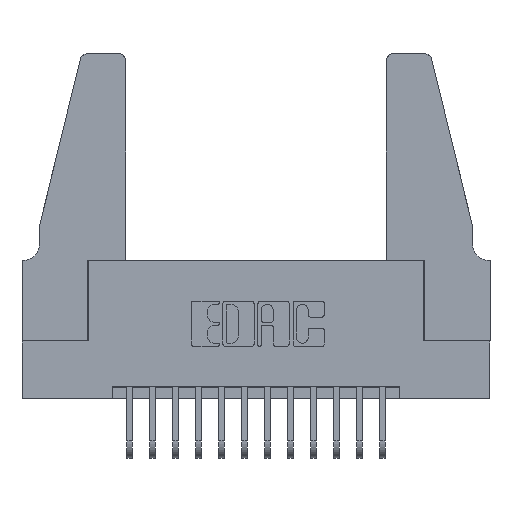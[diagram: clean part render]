
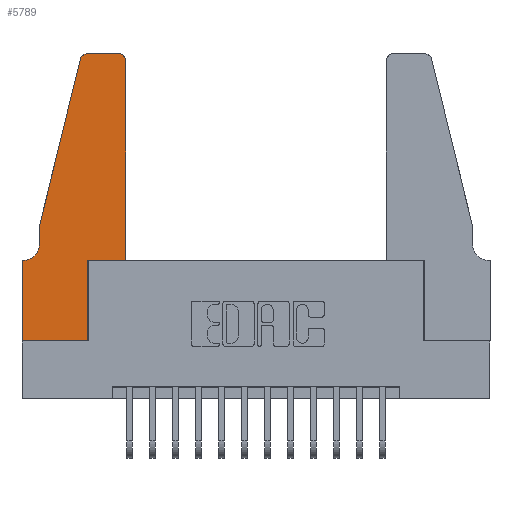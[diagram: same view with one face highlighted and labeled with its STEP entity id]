
A CAD part, top view. The second image highlights one B-rep face of the part: STEP entity #5789.
In plain terms, the highlighted planar face has unit normal (0, 0, 1).
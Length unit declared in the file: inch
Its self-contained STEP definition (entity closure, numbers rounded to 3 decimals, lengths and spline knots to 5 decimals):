
#34 = CARTESIAN_POINT ( 'NONE',  ( 0.4205, 1.22, 0.37 ) ) ;
#195 = EDGE_CURVE ( 'NONE', #236, #10536, #16336, .T. ) ;
#236 = VERTEX_POINT ( 'NONE', #4721 ) ;
#708 = ORIENTED_EDGE ( 'NONE', *, *, #14038, .T. ) ;
#716 = EDGE_CURVE ( 'NONE', #9279, #2787, #15521, .T. ) ;
#988 = EDGE_CURVE ( 'NONE', #12800, #6573, #12059, .T. ) ;
#1186 = DIRECTION ( 'NONE',  ( 0., 1., 0. ) ) ;
#1189 = CARTESIAN_POINT ( 'NONE',  ( 0.0755, 0.5, 0.37 ) ) ;
#1417 = DIRECTION ( 'NONE',  ( 1., 0., 0. ) ) ;
#1573 = CARTESIAN_POINT ( 'NONE',  ( 0., 0., 0.37 ) ) ;
#1578 = CARTESIAN_POINT ( 'NONE',  ( 0.284, 1.22, 0.37 ) ) ;
#1731 = LINE ( 'NONE', #1573, #8723 ) ;
#1789 = DIRECTION ( 'NONE',  ( 0., -1., 0. ) ) ;
#1883 = VECTOR ( 'NONE', #7935, 39.37008 ) ;
#2239 = ORIENTED_EDGE ( 'NONE', *, *, #7657, .T. ) ;
#2275 = EDGE_CURVE ( 'NONE', #6573, #14559, #14823, .T. ) ;
#2377 = FACE_OUTER_BOUND ( 'NONE', #6181, .T. ) ;
#2787 = VERTEX_POINT ( 'NONE', #11949 ) ;
#2985 = DIRECTION ( 'NONE',  ( 0., -1., 0. ) ) ;
#2988 = DIRECTION ( 'NONE',  ( 1., 0., 0. ) ) ;
#3435 = EDGE_CURVE ( 'NONE', #17210, #11579, #15969, .T. ) ;
#3526 = PLANE ( 'NONE',  #13169 ) ;
#3798 = DIRECTION ( 'NONE',  ( 1., 0., 0. ) ) ;
#4721 = CARTESIAN_POINT ( 'NONE',  ( 0.0755, 0.42, 0.37 ) ) ;
#4843 = DIRECTION ( 'NONE',  ( 0., 0., -1. ) ) ;
#4886 = CARTESIAN_POINT ( 'NONE',  ( 0.0055, 0.42, 0.37 ) ) ;
#4916 = VERTEX_POINT ( 'NONE', #16343 ) ;
#4931 = DIRECTION ( 'NONE',  ( 0., 0., 1. ) ) ;
#5191 = DIRECTION ( 'NONE',  ( -1., 0., 0. ) ) ;
#5255 = CARTESIAN_POINT ( 'NONE',  ( 0.4505, 1.22, 0.37 ) ) ;
#5608 = LINE ( 'NONE', #16929, #1883 ) ;
#5740 = CARTESIAN_POINT ( 'NONE',  ( 0.4205, 1.25, 0.37 ) ) ;
#5789 = ADVANCED_FACE ( 'NONE', ( #2377 ), #3526, .T. ) ;
#6181 = EDGE_LOOP ( 'NONE', ( #15195, #12189, #9197, #2239, #9609, #16388, #10016, #13382, #10435, #7247, #10819, #708 ) ) ;
#6261 = CARTESIAN_POINT ( 'NONE',  ( 0., 0.35, 0.37 ) ) ;
#6550 = CIRCLE ( 'NONE', #13140, 0.03 ) ;
#6573 = VERTEX_POINT ( 'NONE', #16811 ) ;
#6599 = CARTESIAN_POINT ( 'NONE',  ( 0., 0., 0.37 ) ) ;
#6627 = VECTOR ( 'NONE', #14822, 39.37008 ) ;
#6824 = DIRECTION ( 'NONE',  ( -0.239, -0.971, 0. ) ) ;
#6870 = CARTESIAN_POINT ( 'NONE',  ( 0., 0., 0.37 ) ) ;
#6939 = EDGE_CURVE ( 'NONE', #2787, #4916, #10712, .T. ) ;
#7191 = LINE ( 'NONE', #17166, #13725 ) ;
#7247 = ORIENTED_EDGE ( 'NONE', *, *, #988, .T. ) ;
#7657 = EDGE_CURVE ( 'NONE', #11044, #236, #10343, .T. ) ;
#7935 = DIRECTION ( 'NONE',  ( -1., 0., 0. ) ) ;
#8176 = VECTOR ( 'NONE', #11530, 39.37008 ) ;
#8723 = VECTOR ( 'NONE', #2985, 39.37008 ) ;
#9197 = ORIENTED_EDGE ( 'NONE', *, *, #9750, .T. ) ;
#9279 = VERTEX_POINT ( 'NONE', #5740 ) ;
#9481 = VERTEX_POINT ( 'NONE', #12821 ) ;
#9609 = ORIENTED_EDGE ( 'NONE', *, *, #195, .T. ) ;
#9732 = DIRECTION ( 'NONE',  ( 0., 0., 1. ) ) ;
#9750 = EDGE_CURVE ( 'NONE', #4916, #11044, #13837, .T. ) ;
#10016 = ORIENTED_EDGE ( 'NONE', *, *, #13219, .T. ) ;
#10085 = CARTESIAN_POINT ( 'NONE',  ( 0.0755, 0.5, 0.37 ) ) ;
#10343 = LINE ( 'NONE', #10085, #16716 ) ;
#10435 = ORIENTED_EDGE ( 'NONE', *, *, #13543, .T. ) ;
#10484 = VECTOR ( 'NONE', #6824, 39.37008 ) ;
#10536 = VERTEX_POINT ( 'NONE', #15200 ) ;
#10712 = CIRCLE ( 'NONE', #12226, 0.03 ) ;
#10819 = ORIENTED_EDGE ( 'NONE', *, *, #2275, .T. ) ;
#10898 = AXIS2_PLACEMENT_3D ( 'NONE', #4886, #4843, #5191 ) ;
#11044 = VERTEX_POINT ( 'NONE', #13102 ) ;
#11149 = DIRECTION ( 'NONE',  ( 0., 0., 1. ) ) ;
#11530 = DIRECTION ( 'NONE',  ( 1., 0., 0. ) ) ;
#11579 = VERTEX_POINT ( 'NONE', #11647 ) ;
#11647 = CARTESIAN_POINT ( 'NONE',  ( 0.2865, 0., 0.37 ) ) ;
#11657 = CARTESIAN_POINT ( 'NONE',  ( 0.4505, 0.35, 0.37 ) ) ;
#11949 = CARTESIAN_POINT ( 'NONE',  ( 0.284, 1.25, 0.37 ) ) ;
#12059 = LINE ( 'NONE', #11657, #8176 ) ;
#12189 = ORIENTED_EDGE ( 'NONE', *, *, #6939, .T. ) ;
#12226 = AXIS2_PLACEMENT_3D ( 'NONE', #1578, #11149, #2988 ) ;
#12252 = CARTESIAN_POINT ( 'NONE',  ( 0.4505, 0.35, 0.37 ) ) ;
#12800 = VERTEX_POINT ( 'NONE', #12881 ) ;
#12821 = CARTESIAN_POINT ( 'NONE',  ( 0., 0.35, 0.37 ) ) ;
#12881 = CARTESIAN_POINT ( 'NONE',  ( 0.2865, 0.35, 0.37 ) ) ;
#13102 = CARTESIAN_POINT ( 'NONE',  ( 0.0755, 0.5, 0.37 ) ) ;
#13140 = AXIS2_PLACEMENT_3D ( 'NONE', #34, #9732, #1417 ) ;
#13169 = AXIS2_PLACEMENT_3D ( 'NONE', #6261, #4931, #14198 ) ;
#13219 = EDGE_CURVE ( 'NONE', #9481, #17210, #1731, .T. ) ;
#13382 = ORIENTED_EDGE ( 'NONE', *, *, #3435, .T. ) ;
#13543 = EDGE_CURVE ( 'NONE', #11579, #12800, #7191, .T. ) ;
#13725 = VECTOR ( 'NONE', #1186, 39.37008 ) ;
#13837 = LINE ( 'NONE', #1189, #10484 ) ;
#14038 = EDGE_CURVE ( 'NONE', #14559, #9279, #6550, .T. ) ;
#14198 = DIRECTION ( 'NONE',  ( 1., 0., 0. ) ) ;
#14559 = VERTEX_POINT ( 'NONE', #5255 ) ;
#14822 = DIRECTION ( 'NONE',  ( 0., 1., 0. ) ) ;
#14823 = LINE ( 'NONE', #12252, #6627 ) ;
#14889 = DIRECTION ( 'NONE',  ( -1., 0., 0. ) ) ;
#15120 = VECTOR ( 'NONE', #14889, 39.37008 ) ;
#15195 = ORIENTED_EDGE ( 'NONE', *, *, #716, .T. ) ;
#15200 = CARTESIAN_POINT ( 'NONE',  ( 0.0055, 0.35, 0.37 ) ) ;
#15521 = LINE ( 'NONE', #15669, #15120 ) ;
#15669 = CARTESIAN_POINT ( 'NONE',  ( 0.2605, 1.25, 0.37 ) ) ;
#15824 = EDGE_CURVE ( 'NONE', #10536, #9481, #5608, .T. ) ;
#15969 = LINE ( 'NONE', #6599, #16370 ) ;
#16336 = CIRCLE ( 'NONE', #10898, 0.07 ) ;
#16343 = CARTESIAN_POINT ( 'NONE',  ( 0.25487, 1.22718, 0.37 ) ) ;
#16370 = VECTOR ( 'NONE', #3798, 39.37008 ) ;
#16388 = ORIENTED_EDGE ( 'NONE', *, *, #15824, .T. ) ;
#16716 = VECTOR ( 'NONE', #1789, 39.37008 ) ;
#16811 = CARTESIAN_POINT ( 'NONE',  ( 0.4505, 0.35, 0.37 ) ) ;
#16929 = CARTESIAN_POINT ( 'NONE',  ( 0.0755, 0.35, 0.37 ) ) ;
#17166 = CARTESIAN_POINT ( 'NONE',  ( 0.2865, 0.35, 0.37 ) ) ;
#17210 = VERTEX_POINT ( 'NONE', #6870 ) ;
